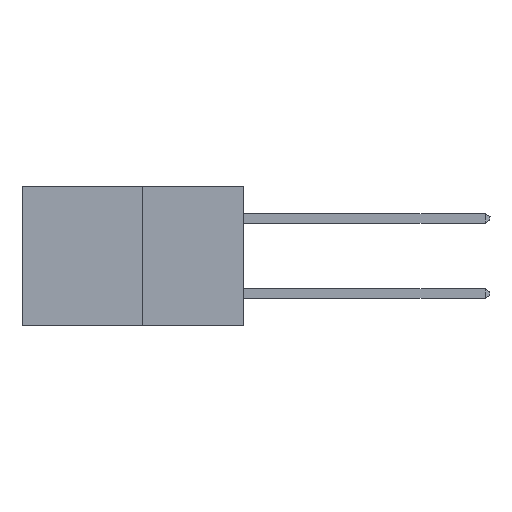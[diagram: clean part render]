
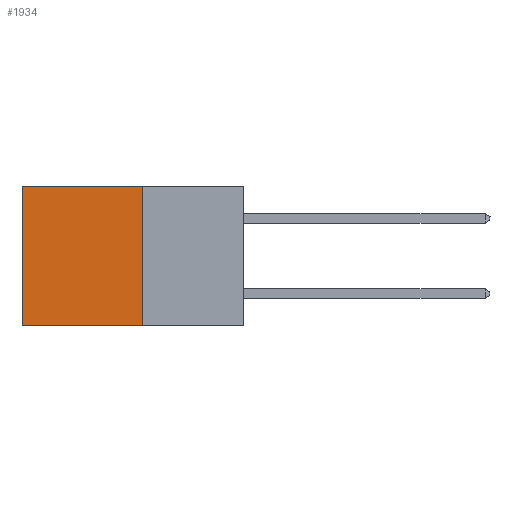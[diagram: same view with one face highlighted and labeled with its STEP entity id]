
A CAD part, left-side view. The second image highlights one B-rep face of the part: STEP entity #1934.
In plain terms, the highlighted planar face has unit normal (-1, 0, 0).
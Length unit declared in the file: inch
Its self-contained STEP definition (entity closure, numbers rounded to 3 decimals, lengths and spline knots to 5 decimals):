
#1251 = EDGE_LOOP ( 'NONE', ( #27563, #2880, #24782, #13145 ) ) ;
#1934 = ADVANCED_FACE ( 'NONE', ( #10360 ), #15340, .F. ) ;
#2237 = CARTESIAN_POINT ( 'NONE',  ( 0.277, 0.27, -0.37 ) ) ;
#2880 = ORIENTED_EDGE ( 'NONE', *, *, #22794, .F. ) ;
#4182 = VECTOR ( 'NONE', #12321, 39.37008 ) ;
#4836 = CARTESIAN_POINT ( 'NONE',  ( 0.277, 0.59, 0. ) ) ;
#6115 = CARTESIAN_POINT ( 'NONE',  ( 0.277, 0.27, 0. ) ) ;
#7050 = CARTESIAN_POINT ( 'NONE',  ( 0.277, 0.27, -0.37 ) ) ;
#10223 = CARTESIAN_POINT ( 'NONE',  ( 0.277, 0.27, -0.37 ) ) ;
#10360 = FACE_OUTER_BOUND ( 'NONE', #1251, .T. ) ;
#11197 = CARTESIAN_POINT ( 'NONE',  ( 0.277, 0.59, -0.37 ) ) ;
#11351 = LINE ( 'NONE', #7050, #4182 ) ;
#12321 = DIRECTION ( 'NONE',  ( 0., 1., 0. ) ) ;
#12705 = VERTEX_POINT ( 'NONE', #4836 ) ;
#13145 = ORIENTED_EDGE ( 'NONE', *, *, #27561, .T. ) ;
#14422 = VECTOR ( 'NONE', #32042, 39.37008 ) ;
#14657 = DIRECTION ( 'NONE',  ( 0., 1., 0. ) ) ;
#14807 = VERTEX_POINT ( 'NONE', #17657 ) ;
#14929 = EDGE_CURVE ( 'NONE', #15823, #19433, #22487, .T. ) ;
#15340 = PLANE ( 'NONE',  #33602 ) ;
#15823 = VERTEX_POINT ( 'NONE', #6115 ) ;
#17657 = CARTESIAN_POINT ( 'NONE',  ( 0.277, 0.59, -0.37 ) ) ;
#19433 = VERTEX_POINT ( 'NONE', #25251 ) ;
#20812 = DIRECTION ( 'NONE',  ( 0., 0., -1. ) ) ;
#20901 = VECTOR ( 'NONE', #14657, 39.37008 ) ;
#21708 = LINE ( 'NONE', #27549, #20901 ) ;
#22487 = LINE ( 'NONE', #2237, #29381 ) ;
#22794 = EDGE_CURVE ( 'NONE', #19433, #14807, #11351, .T. ) ;
#24782 = ORIENTED_EDGE ( 'NONE', *, *, #14929, .F. ) ;
#25251 = CARTESIAN_POINT ( 'NONE',  ( 0.277, 0.27, -0.37 ) ) ;
#27357 = EDGE_CURVE ( 'NONE', #12705, #14807, #28176, .T. ) ;
#27549 = CARTESIAN_POINT ( 'NONE',  ( 0.277, 0.27, 0. ) ) ;
#27561 = EDGE_CURVE ( 'NONE', #15823, #12705, #21708, .T. ) ;
#27563 = ORIENTED_EDGE ( 'NONE', *, *, #27357, .T. ) ;
#28176 = LINE ( 'NONE', #11197, #14422 ) ;
#29381 = VECTOR ( 'NONE', #20812, 39.37008 ) ;
#32042 = DIRECTION ( 'NONE',  ( 0., 0., -1. ) ) ;
#32355 = DIRECTION ( 'NONE',  ( 0., 0., -1. ) ) ;
#32398 = DIRECTION ( 'NONE',  ( 1., 0., 0. ) ) ;
#33602 = AXIS2_PLACEMENT_3D ( 'NONE', #10223, #32398, #32355 ) ;
